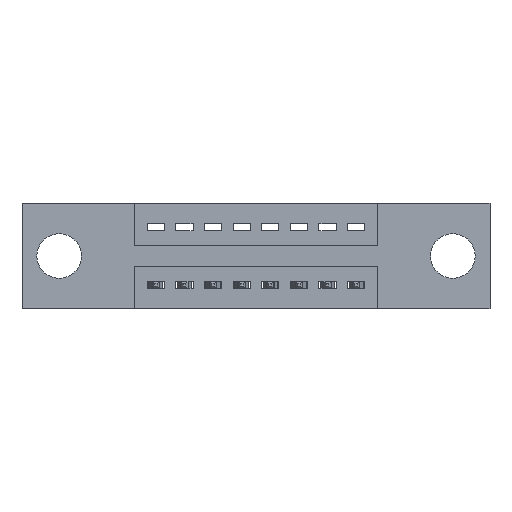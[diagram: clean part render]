
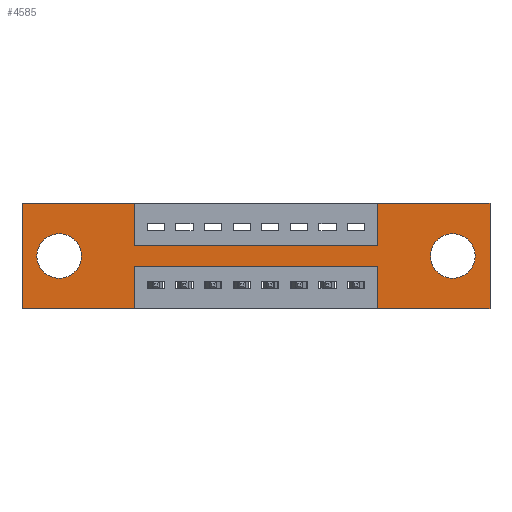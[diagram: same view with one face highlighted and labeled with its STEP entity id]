
A CAD part, front view. The second image highlights one B-rep face of the part: STEP entity #4585.
In plain terms, the highlighted planar face has unit normal (0, -1, 0).
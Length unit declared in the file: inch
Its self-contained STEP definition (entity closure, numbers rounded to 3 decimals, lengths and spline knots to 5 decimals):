
#71 = VERTEX_POINT ( 'NONE', #3504 ) ;
#91 = VERTEX_POINT ( 'NONE', #4838 ) ;
#209 = EDGE_CURVE ( 'NONE', #946, #9417, #8069, .T. ) ;
#251 = LINE ( 'NONE', #7537, #6944 ) ;
#270 = VECTOR ( 'NONE', #10285, 39.37008 ) ;
#503 = VECTOR ( 'NONE', #9908, 39.37008 ) ;
#586 = ORIENTED_EDGE ( 'NONE', *, *, #4640, .T. ) ;
#598 = ORIENTED_EDGE ( 'NONE', *, *, #5790, .T. ) ;
#608 = ORIENTED_EDGE ( 'NONE', *, *, #5923, .T. ) ;
#613 = EDGE_CURVE ( 'NONE', #7586, #732, #2670, .T. ) ;
#622 = ORIENTED_EDGE ( 'NONE', *, *, #10620, .T. ) ;
#629 = DIRECTION ( 'NONE',  ( 0., 0., 1. ) ) ;
#635 = ORIENTED_EDGE ( 'NONE', *, *, #1198, .F. ) ;
#645 = ORIENTED_EDGE ( 'NONE', *, *, #6751, .F. ) ;
#654 = ORIENTED_EDGE ( 'NONE', *, *, #8915, .F. ) ;
#666 = ORIENTED_EDGE ( 'NONE', *, *, #209, .F. ) ;
#672 = ORIENTED_EDGE ( 'NONE', *, *, #6155, .F. ) ;
#732 = VERTEX_POINT ( 'NONE', #9033 ) ;
#750 = ORIENTED_EDGE ( 'NONE', *, *, #10009, .F. ) ;
#754 = CARTESIAN_POINT ( 'NONE',  ( 0., 0., -0.37 ) ) ;
#827 = CARTESIAN_POINT ( 'NONE',  ( 0., 0., 0. ) ) ;
#879 = ORIENTED_EDGE ( 'NONE', *, *, #7360, .F. ) ;
#884 = ORIENTED_EDGE ( 'NONE', *, *, #7878, .F. ) ;
#896 = ORIENTED_EDGE ( 'NONE', *, *, #8421, .F. ) ;
#904 = ORIENTED_EDGE ( 'NONE', *, *, #2366, .F. ) ;
#927 = ORIENTED_EDGE ( 'NONE', *, *, #613, .F. ) ;
#940 = ORIENTED_EDGE ( 'NONE', *, *, #5132, .F. ) ;
#946 = VERTEX_POINT ( 'NONE', #1010 ) ;
#1010 = CARTESIAN_POINT ( 'NONE',  ( 1.635, 0., -0.37 ) ) ;
#1047 = CARTESIAN_POINT ( 'NONE',  ( 0.13, 0., -0.185 ) ) ;
#1069 = AXIS2_PLACEMENT_3D ( 'NONE', #8553, #3587, #9260 ) ;
#1157 = DIRECTION ( 'NONE',  ( 0., 0., -1. ) ) ;
#1172 = DIRECTION ( 'NONE',  ( 0., -1., 0. ) ) ;
#1198 = EDGE_CURVE ( 'NONE', #91, #6533, #1561, .T. ) ;
#1558 = CARTESIAN_POINT ( 'NONE',  ( 0., 0., 0. ) ) ;
#1561 = LINE ( 'NONE', #8760, #10176 ) ;
#1619 = VECTOR ( 'NONE', #4244, 39.37008 ) ;
#1884 = DIRECTION ( 'NONE',  ( 0., 0., -1. ) ) ;
#1887 = DIRECTION ( 'NONE',  ( 0., 1., 0. ) ) ;
#1902 = CARTESIAN_POINT ( 'NONE',  ( 1.505, 0., -0.185 ) ) ;
#1970 = DIRECTION ( 'NONE',  ( 0., 0., 1. ) ) ;
#2066 = VECTOR ( 'NONE', #8659, 39.37008 ) ;
#2280 = DIRECTION ( 'NONE',  ( 0., 0., -1. ) ) ;
#2366 = EDGE_CURVE ( 'NONE', #732, #3863, #6365, .T. ) ;
#2371 = VECTOR ( 'NONE', #2280, 39.37008 ) ;
#2670 = LINE ( 'NONE', #827, #270 ) ;
#2833 = CARTESIAN_POINT ( 'NONE',  ( 1.2425, 0., -0.22 ) ) ;
#3011 = VERTEX_POINT ( 'NONE', #3813 ) ;
#3504 = CARTESIAN_POINT ( 'NONE',  ( 0.13, 0., -0.107 ) ) ;
#3587 = DIRECTION ( 'NONE',  ( 0., 1., 0. ) ) ;
#3706 = VECTOR ( 'NONE', #9543, 39.37008 ) ;
#3734 = CARTESIAN_POINT ( 'NONE',  ( 0.3925, 0., -0.15 ) ) ;
#3768 = EDGE_LOOP ( 'NONE', ( #608, #622 ) ) ;
#3785 = DIRECTION ( 'NONE',  ( 1., 0., 0. ) ) ;
#3813 = CARTESIAN_POINT ( 'NONE',  ( 0.3925, 0., -0.15 ) ) ;
#3829 = PLANE ( 'NONE',  #6938 ) ;
#3846 = CARTESIAN_POINT ( 'NONE',  ( 0., 0., 0. ) ) ;
#3863 = VERTEX_POINT ( 'NONE', #6818 ) ;
#4005 = LINE ( 'NONE', #7269, #3706 ) ;
#4078 = AXIS2_PLACEMENT_3D ( 'NONE', #1047, #7081, #1970 ) ;
#4083 = VERTEX_POINT ( 'NONE', #6324 ) ;
#4244 = DIRECTION ( 'NONE',  ( 1., 0., 0. ) ) ;
#4261 = LINE ( 'NONE', #1558, #1619 ) ;
#4293 = CARTESIAN_POINT ( 'NONE',  ( 1.635, 0., 0. ) ) ;
#4414 = LINE ( 'NONE', #3734, #10350 ) ;
#4585 = ADVANCED_FACE ( 'NONE', ( #7319, #9108, #7050 ), #3829, .T. ) ;
#4640 = EDGE_CURVE ( 'NONE', #8880, #9489, #8670, .T. ) ;
#4728 = LINE ( 'NONE', #8151, #2371 ) ;
#4838 = CARTESIAN_POINT ( 'NONE',  ( 0.3925, 0., -0.22 ) ) ;
#4964 = VERTEX_POINT ( 'NONE', #7924 ) ;
#5121 = CIRCLE ( 'NONE', #4078, 0.078 ) ;
#5132 = EDGE_CURVE ( 'NONE', #6533, #7586, #251, .T. ) ;
#5503 = CARTESIAN_POINT ( 'NONE',  ( 0., 0., -0.37 ) ) ;
#5790 = EDGE_CURVE ( 'NONE', #9489, #8880, #5938, .T. ) ;
#5923 = EDGE_CURVE ( 'NONE', #71, #8280, #5121, .T. ) ;
#5925 = DIRECTION ( 'NONE',  ( 0., 1., 0. ) ) ;
#5938 = CIRCLE ( 'NONE', #1069, 0.078 ) ;
#6044 = LINE ( 'NONE', #6382, #9625 ) ;
#6155 = EDGE_CURVE ( 'NONE', #8162, #946, #4728, .T. ) ;
#6164 = DIRECTION ( 'NONE',  ( -1., 0., 0. ) ) ;
#6324 = CARTESIAN_POINT ( 'NONE',  ( 1.2425, 0., -0.15 ) ) ;
#6365 = LINE ( 'NONE', #3846, #9907 ) ;
#6382 = CARTESIAN_POINT ( 'NONE',  ( 0.3925, 0., 0. ) ) ;
#6533 = VERTEX_POINT ( 'NONE', #10222 ) ;
#6751 = EDGE_CURVE ( 'NONE', #7239, #91, #7415, .T. ) ;
#6818 = CARTESIAN_POINT ( 'NONE',  ( 0.3925, 0., 0. ) ) ;
#6850 = CARTESIAN_POINT ( 'NONE',  ( 0., 0., -0.37 ) ) ;
#6936 = CARTESIAN_POINT ( 'NONE',  ( 0.13, 0., -0.263 ) ) ;
#6938 = AXIS2_PLACEMENT_3D ( 'NONE', #754, #1172, #1157 ) ;
#6944 = VECTOR ( 'NONE', #7072, 39.37008 ) ;
#7050 = FACE_OUTER_BOUND ( 'NONE', #8417, .T. ) ;
#7072 = DIRECTION ( 'NONE',  ( -1., 0., 0. ) ) ;
#7081 = DIRECTION ( 'NONE',  ( 0., 1., 0. ) ) ;
#7111 = DIRECTION ( 'NONE',  ( 1., 0., 0. ) ) ;
#7239 = VERTEX_POINT ( 'NONE', #2833 ) ;
#7269 = CARTESIAN_POINT ( 'NONE',  ( 1.2425, 0., 0. ) ) ;
#7319 = FACE_BOUND ( 'NONE', #9902, .T. ) ;
#7360 = EDGE_CURVE ( 'NONE', #4083, #4964, #4005, .T. ) ;
#7415 = LINE ( 'NONE', #9180, #503 ) ;
#7537 = CARTESIAN_POINT ( 'NONE',  ( 0., 0., -0.37 ) ) ;
#7586 = VERTEX_POINT ( 'NONE', #6850 ) ;
#7665 = DIRECTION ( 'NONE',  ( 0., 0., -1. ) ) ;
#7858 = CARTESIAN_POINT ( 'NONE',  ( 1.2425, 0., -0.37 ) ) ;
#7878 = EDGE_CURVE ( 'NONE', #3011, #4083, #4414, .T. ) ;
#7924 = CARTESIAN_POINT ( 'NONE',  ( 1.2425, 0., 0. ) ) ;
#8001 = AXIS2_PLACEMENT_3D ( 'NONE', #1902, #1887, #1884 ) ;
#8069 = LINE ( 'NONE', #5503, #10430 ) ;
#8151 = CARTESIAN_POINT ( 'NONE',  ( 1.635, 0., 0. ) ) ;
#8162 = VERTEX_POINT ( 'NONE', #4293 ) ;
#8280 = VERTEX_POINT ( 'NONE', #6936 ) ;
#8417 = EDGE_LOOP ( 'NONE', ( #635, #645, #654, #666, #672, #750, #879, #884, #896, #904, #927, #940 ) ) ;
#8421 = EDGE_CURVE ( 'NONE', #3863, #3011, #6044, .T. ) ;
#8553 = CARTESIAN_POINT ( 'NONE',  ( 1.505, 0., -0.185 ) ) ;
#8659 = DIRECTION ( 'NONE',  ( 0., 0., 1. ) ) ;
#8670 = CIRCLE ( 'NONE', #8001, 0.078 ) ;
#8707 = CIRCLE ( 'NONE', #10320, 0.078 ) ;
#8760 = CARTESIAN_POINT ( 'NONE',  ( 0.3925, 0., -0.37 ) ) ;
#8880 = VERTEX_POINT ( 'NONE', #9290 ) ;
#8915 = EDGE_CURVE ( 'NONE', #9417, #7239, #9176, .T. ) ;
#9033 = CARTESIAN_POINT ( 'NONE',  ( 0., 0., 0. ) ) ;
#9108 = FACE_BOUND ( 'NONE', #3768, .T. ) ;
#9176 = LINE ( 'NONE', #7858, #2066 ) ;
#9180 = CARTESIAN_POINT ( 'NONE',  ( 0.3925, 0., -0.22 ) ) ;
#9260 = DIRECTION ( 'NONE',  ( 0., 0., -1. ) ) ;
#9290 = CARTESIAN_POINT ( 'NONE',  ( 1.505, 0., -0.107 ) ) ;
#9417 = VERTEX_POINT ( 'NONE', #10549 ) ;
#9461 = DIRECTION ( 'NONE',  ( 0., 0., -1. ) ) ;
#9489 = VERTEX_POINT ( 'NONE', #10581 ) ;
#9543 = DIRECTION ( 'NONE',  ( 0., 0., 1. ) ) ;
#9625 = VECTOR ( 'NONE', #9461, 39.37008 ) ;
#9902 = EDGE_LOOP ( 'NONE', ( #586, #598 ) ) ;
#9907 = VECTOR ( 'NONE', #3785, 39.37008 ) ;
#9908 = DIRECTION ( 'NONE',  ( -1., 0., 0. ) ) ;
#10009 = EDGE_CURVE ( 'NONE', #4964, #8162, #4261, .T. ) ;
#10176 = VECTOR ( 'NONE', #7665, 39.37008 ) ;
#10222 = CARTESIAN_POINT ( 'NONE',  ( 0.3925, 0., -0.37 ) ) ;
#10285 = DIRECTION ( 'NONE',  ( 0., 0., 1. ) ) ;
#10320 = AXIS2_PLACEMENT_3D ( 'NONE', #10425, #5925, #629 ) ;
#10350 = VECTOR ( 'NONE', #7111, 39.37008 ) ;
#10425 = CARTESIAN_POINT ( 'NONE',  ( 0.13, 0., -0.185 ) ) ;
#10430 = VECTOR ( 'NONE', #6164, 39.37008 ) ;
#10549 = CARTESIAN_POINT ( 'NONE',  ( 1.2425, 0., -0.37 ) ) ;
#10581 = CARTESIAN_POINT ( 'NONE',  ( 1.505, 0., -0.263 ) ) ;
#10620 = EDGE_CURVE ( 'NONE', #8280, #71, #8707, .T. ) ;
